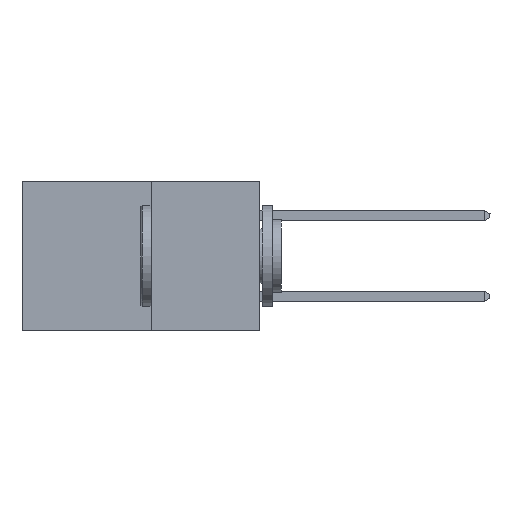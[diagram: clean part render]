
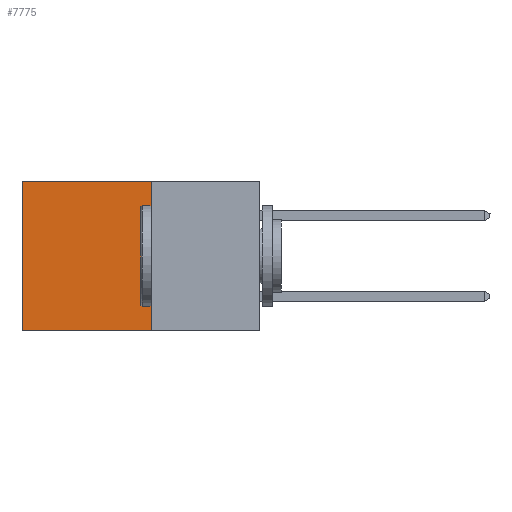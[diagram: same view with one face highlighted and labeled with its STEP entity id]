
A CAD part, left-side view. The second image highlights one B-rep face of the part: STEP entity #7775.
In plain terms, the highlighted planar face has unit normal (-1, 0, 0).
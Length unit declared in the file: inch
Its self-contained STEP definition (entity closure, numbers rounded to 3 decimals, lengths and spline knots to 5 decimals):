
#22 = EDGE_LOOP ( 'NONE', ( #16407, #8029, #9572, #11198 ) ) ;
#207 = AXIS2_PLACEMENT_3D ( 'NONE', #16532, #15782, #15648 ) ;
#285 = DIRECTION ( 'NONE',  ( 0., 1., 0. ) ) ;
#456 = CARTESIAN_POINT ( 'NONE',  ( 0.277, 0.27, 0. ) ) ;
#619 = PLANE ( 'NONE',  #207 ) ;
#3233 = DIRECTION ( 'NONE',  ( 0., 1., 0. ) ) ;
#5035 = FACE_OUTER_BOUND ( 'NONE', #22, .T. ) ;
#5923 = CARTESIAN_POINT ( 'NONE',  ( 0.277, 0.27, -0.37 ) ) ;
#5980 = VECTOR ( 'NONE', #12111, 39.37008 ) ;
#6039 = EDGE_CURVE ( 'NONE', #8444, #10325, #13986, .T. ) ;
#6703 = VERTEX_POINT ( 'NONE', #13781 ) ;
#6704 = DIRECTION ( 'NONE',  ( 0., 0., -1. ) ) ;
#6726 = CARTESIAN_POINT ( 'NONE',  ( 0.277, 0.59, -0.37 ) ) ;
#6845 = CARTESIAN_POINT ( 'NONE',  ( 0.277, 0.59, 0. ) ) ;
#7153 = EDGE_CURVE ( 'NONE', #10325, #6703, #16758, .T. ) ;
#7254 = VECTOR ( 'NONE', #3233, 39.37008 ) ;
#7775 = ADVANCED_FACE ( 'NONE', ( #5035 ), #619, .F. ) ;
#8029 = ORIENTED_EDGE ( 'NONE', *, *, #13484, .F. ) ;
#8324 = CARTESIAN_POINT ( 'NONE',  ( 0.277, 0.27, 0. ) ) ;
#8444 = VERTEX_POINT ( 'NONE', #8324 ) ;
#9572 = ORIENTED_EDGE ( 'NONE', *, *, #16739, .F. ) ;
#10325 = VERTEX_POINT ( 'NONE', #6845 ) ;
#10660 = VECTOR ( 'NONE', #6704, 39.37008 ) ;
#10923 = VERTEX_POINT ( 'NONE', #16727 ) ;
#11198 = ORIENTED_EDGE ( 'NONE', *, *, #6039, .T. ) ;
#12111 = DIRECTION ( 'NONE',  ( 0., 0., -1. ) ) ;
#12905 = LINE ( 'NONE', #15619, #5980 ) ;
#13484 = EDGE_CURVE ( 'NONE', #10923, #6703, #14168, .T. ) ;
#13574 = VECTOR ( 'NONE', #285, 39.37008 ) ;
#13781 = CARTESIAN_POINT ( 'NONE',  ( 0.277, 0.59, -0.37 ) ) ;
#13986 = LINE ( 'NONE', #456, #13574 ) ;
#14168 = LINE ( 'NONE', #5923, #7254 ) ;
#15619 = CARTESIAN_POINT ( 'NONE',  ( 0.277, 0.27, -0.37 ) ) ;
#15648 = DIRECTION ( 'NONE',  ( 0., 0., -1. ) ) ;
#15782 = DIRECTION ( 'NONE',  ( 1., 0., 0. ) ) ;
#16407 = ORIENTED_EDGE ( 'NONE', *, *, #7153, .T. ) ;
#16532 = CARTESIAN_POINT ( 'NONE',  ( 0.277, 0.27, -0.37 ) ) ;
#16727 = CARTESIAN_POINT ( 'NONE',  ( 0.277, 0.27, -0.37 ) ) ;
#16739 = EDGE_CURVE ( 'NONE', #8444, #10923, #12905, .T. ) ;
#16758 = LINE ( 'NONE', #6726, #10660 ) ;
